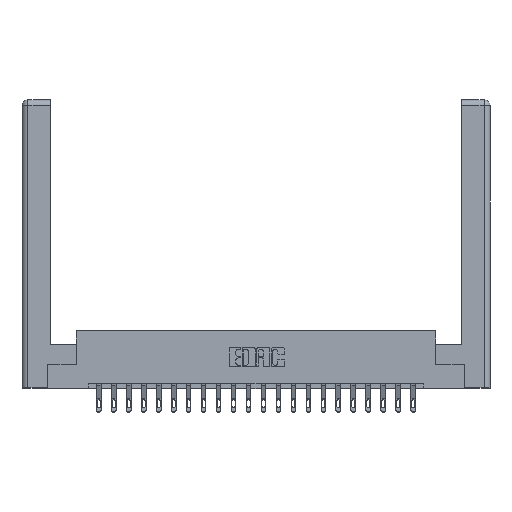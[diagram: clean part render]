
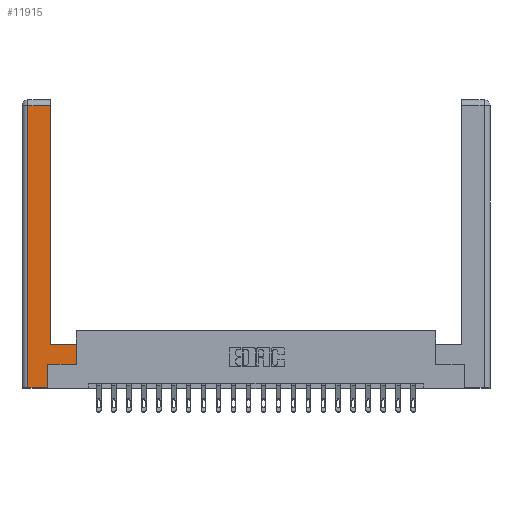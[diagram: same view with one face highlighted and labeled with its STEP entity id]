
A CAD part, top view. The second image highlights one B-rep face of the part: STEP entity #11915.
In plain terms, the highlighted planar face has unit normal (0, 0, 1).
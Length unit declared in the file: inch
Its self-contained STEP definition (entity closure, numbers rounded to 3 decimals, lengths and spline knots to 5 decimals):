
#40 = EDGE_CURVE ( 'NONE', #6922, #7726, #19495, .T. ) ;
#305 = CARTESIAN_POINT ( 'NONE',  ( 0.565, 0.45, 0. ) ) ;
#533 = DIRECTION ( 'NONE',  ( -1., 0., 0. ) ) ;
#1156 = LINE ( 'NONE', #305, #19237 ) ;
#1291 = VECTOR ( 'NONE', #1848, 39.37008 ) ;
#1848 = DIRECTION ( 'NONE',  ( 1., 0., 0. ) ) ;
#3172 = EDGE_LOOP ( 'NONE', ( #15948, #17872, #17765, #15194, #15139, #21986, #11587, #12802 ) ) ;
#3217 = VECTOR ( 'NONE', #4903, 39.37008 ) ;
#3623 = FACE_OUTER_BOUND ( 'NONE', #3172, .T. ) ;
#4626 = LINE ( 'NONE', #10838, #9310 ) ;
#4878 = VERTEX_POINT ( 'NONE', #21353 ) ;
#4903 = DIRECTION ( 'NONE',  ( 0., 1., 0. ) ) ;
#5576 = VECTOR ( 'NONE', #15134, 39.37008 ) ;
#5744 = VERTEX_POINT ( 'NONE', #21324 ) ;
#6922 = VERTEX_POINT ( 'NONE', #14430 ) ;
#7322 = DIRECTION ( 'NONE',  ( 0., -1., 0. ) ) ;
#7677 = LINE ( 'NONE', #19360, #8522 ) ;
#7726 = VERTEX_POINT ( 'NONE', #13032 ) ;
#7948 = EDGE_CURVE ( 'NONE', #5744, #4878, #14636, .T. ) ;
#8522 = VECTOR ( 'NONE', #7322, 39.37008 ) ;
#9172 = EDGE_CURVE ( 'NONE', #21423, #6922, #1156, .T. ) ;
#9310 = VECTOR ( 'NONE', #10913, 39.37008 ) ;
#9496 = CARTESIAN_POINT ( 'NONE',  ( 0.295, 0.45, 0. ) ) ;
#10334 = LINE ( 'NONE', #19163, #3217 ) ;
#10462 = EDGE_CURVE ( 'NONE', #7726, #5744, #4626, .T. ) ;
#10838 = CARTESIAN_POINT ( 'NONE',  ( 0.295, 3., 0. ) ) ;
#10913 = DIRECTION ( 'NONE',  ( 0., 1., 0. ) ) ;
#11408 = CARTESIAN_POINT ( 'NONE',  ( 0.0615, 2.94, 0. ) ) ;
#11509 = EDGE_CURVE ( 'NONE', #21534, #14323, #10334, .T. ) ;
#11587 = ORIENTED_EDGE ( 'NONE', *, *, #9172, .T. ) ;
#11915 = ADVANCED_FACE ( 'NONE', ( #3623 ), #16297, .F. ) ;
#12802 = ORIENTED_EDGE ( 'NONE', *, *, #40, .T. ) ;
#13032 = CARTESIAN_POINT ( 'NONE',  ( 0.295, 0.45, 0. ) ) ;
#13070 = CARTESIAN_POINT ( 'NONE',  ( 0.565, 0.245, 0. ) ) ;
#14323 = VERTEX_POINT ( 'NONE', #21532 ) ;
#14430 = CARTESIAN_POINT ( 'NONE',  ( 0.565, 0.45, 0. ) ) ;
#14636 = LINE ( 'NONE', #11408, #5576 ) ;
#14676 = EDGE_CURVE ( 'NONE', #21788, #21534, #15537, .T. ) ;
#15134 = DIRECTION ( 'NONE',  ( -1., 0., 0. ) ) ;
#15139 = ORIENTED_EDGE ( 'NONE', *, *, #11509, .T. ) ;
#15194 = ORIENTED_EDGE ( 'NONE', *, *, #14676, .T. ) ;
#15370 = AXIS2_PLACEMENT_3D ( 'NONE', #18049, #21697, #533 ) ;
#15537 = LINE ( 'NONE', #20829, #1291 ) ;
#15798 = CARTESIAN_POINT ( 'NONE',  ( 0.0615, 0., 0. ) ) ;
#15948 = ORIENTED_EDGE ( 'NONE', *, *, #10462, .T. ) ;
#16187 = VECTOR ( 'NONE', #18286, 39.37008 ) ;
#16277 = DIRECTION ( 'NONE',  ( 1., 0., 0. ) ) ;
#16297 = PLANE ( 'NONE',  #15370 ) ;
#16810 = CARTESIAN_POINT ( 'NONE',  ( 0.265, 0., 0. ) ) ;
#17193 = VECTOR ( 'NONE', #16277, 39.37008 ) ;
#17765 = ORIENTED_EDGE ( 'NONE', *, *, #19626, .T. ) ;
#17872 = ORIENTED_EDGE ( 'NONE', *, *, #7948, .T. ) ;
#18049 = CARTESIAN_POINT ( 'NONE',  ( 0., 0., 0. ) ) ;
#18286 = DIRECTION ( 'NONE',  ( -1., 0., 0. ) ) ;
#19163 = CARTESIAN_POINT ( 'NONE',  ( 0.265, 0.245, 0. ) ) ;
#19237 = VECTOR ( 'NONE', #20948, 39.37008 ) ;
#19360 = CARTESIAN_POINT ( 'NONE',  ( 0.0615, 0., 0. ) ) ;
#19495 = LINE ( 'NONE', #9496, #16187 ) ;
#19585 = CARTESIAN_POINT ( 'NONE',  ( 0.565, 0.245, 0. ) ) ;
#19626 = EDGE_CURVE ( 'NONE', #4878, #21788, #7677, .T. ) ;
#20829 = CARTESIAN_POINT ( 'NONE',  ( 0.265, 0., 0. ) ) ;
#20948 = DIRECTION ( 'NONE',  ( 0., 1., 0. ) ) ;
#21231 = EDGE_CURVE ( 'NONE', #14323, #21423, #21814, .T. ) ;
#21324 = CARTESIAN_POINT ( 'NONE',  ( 0.295, 2.94, 0. ) ) ;
#21353 = CARTESIAN_POINT ( 'NONE',  ( 0.0615, 2.94, 0. ) ) ;
#21423 = VERTEX_POINT ( 'NONE', #13070 ) ;
#21532 = CARTESIAN_POINT ( 'NONE',  ( 0.265, 0.245, 0. ) ) ;
#21534 = VERTEX_POINT ( 'NONE', #16810 ) ;
#21697 = DIRECTION ( 'NONE',  ( 0., 0., -1. ) ) ;
#21788 = VERTEX_POINT ( 'NONE', #15798 ) ;
#21814 = LINE ( 'NONE', #19585, #17193 ) ;
#21986 = ORIENTED_EDGE ( 'NONE', *, *, #21231, .T. ) ;
